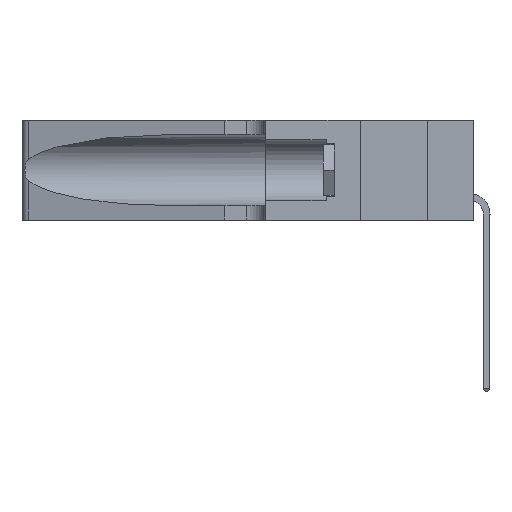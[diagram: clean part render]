
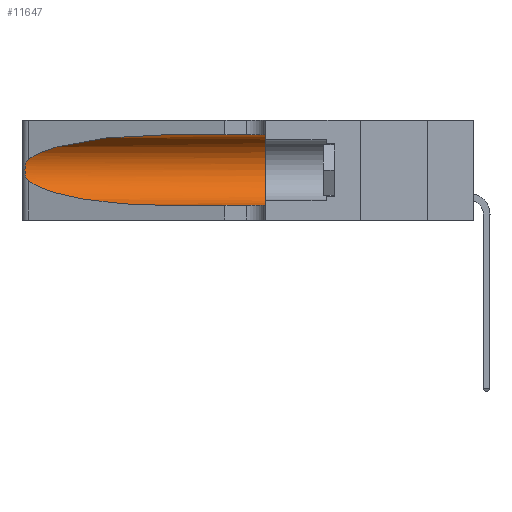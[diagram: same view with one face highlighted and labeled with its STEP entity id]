
A CAD part, left-side view. The second image highlights one B-rep face of the part: STEP entity #11647.
In plain terms, the highlighted cylindrical face has radius 3.308 mm (diameter 6.617 mm), a partial arc.
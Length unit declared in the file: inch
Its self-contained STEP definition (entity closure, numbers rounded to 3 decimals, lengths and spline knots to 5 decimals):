
#360 = EDGE_CURVE ( 'NONE', #12610, #28026, #2224, .T. ) ;
#1036 = CARTESIAN_POINT ( 'NONE',  ( 0.25639, 1.23184, 0.21858 ) ) ;
#2037 = AXIS2_PLACEMENT_3D ( 'NONE', #21559, #14705, #48827 ) ;
#2224 = CIRCLE ( 'NONE', #18384, 0.13025 ) ;
#2693 = CARTESIAN_POINT ( 'NONE',  ( 0.2373, 1.15595, 0.28018 ) ) ;
#3756 = VERTEX_POINT ( 'NONE', #14707 ) ;
#6056 = FACE_OUTER_BOUND ( 'NONE', #37666, .T. ) ;
#6677 = CARTESIAN_POINT ( 'NONE',  ( 0.18966, 0.96281, 0.31525 ) ) ;
#8108 = EDGE_CURVE ( 'NONE', #3756, #28026, #24553, .T. ) ;
#8240 = CARTESIAN_POINT ( 'NONE',  ( 0.25639, 1.23186, 0.15144 ) ) ;
#8394 = CARTESIAN_POINT ( 'NONE',  ( 0.1305, 0.35, 0.31525 ) ) ;
#8759 = CARTESIAN_POINT ( 'NONE',  ( 0.2373, 1.15595, 0.08982 ) ) ;
#11647 = ADVANCED_FACE ( 'NONE', ( #6056 ), #13809, .F. ) ;
#11880 = VERTEX_POINT ( 'NONE', #24815 ) ;
#11924 = CARTESIAN_POINT ( 'NONE',  ( 0.25854, 1.2359, 0.20912 ) ) ;
#12003 = DIRECTION ( 'NONE',  ( 0., -1., 0. ) ) ;
#12610 = VERTEX_POINT ( 'NONE', #8394 ) ;
#13329 = ORIENTED_EDGE ( 'NONE', *, *, #45015, .F. ) ;
#13809 = CYLINDRICAL_SURFACE ( 'NONE', #2037, 0.13025 ) ;
#14033 = B_SPLINE_CURVE_WITH_KNOTS ( 'NONE', 3,
 ( #19439, #45797, #1036, #16199, #11924, #20214, #23894, #38654, #46514, #27074, #42968, #8240, #31607, #34956 ),
 .UNSPECIFIED., .F., .F.,
 ( 4, 2, 2, 2, 2, 2, 4 ),
 ( 0., 0.00027, 0.00053, 0.00107, 0.0016, 0.00187, 0.00214 ),
 .UNSPECIFIED. ) ;
#14705 = DIRECTION ( 'NONE',  ( 0., -1., 0. ) ) ;
#14707 = CARTESIAN_POINT ( 'NONE',  ( 0.1305, 0.72297, 0.05475 ) ) ;
#16199 = CARTESIAN_POINT ( 'NONE',  ( 0.25787, 1.23484, 0.2124 ) ) ;
#16673 = CARTESIAN_POINT ( 'NONE',  ( 0.1305, 1.61858, 0.31525 ) ) ;
#18384 = AXIS2_PLACEMENT_3D ( 'NONE', #45486, #45820, #48797 ) ;
#19439 = CARTESIAN_POINT ( 'NONE',  ( 0.25487, 1.22718, 0.22369 ) ) ;
#20214 = CARTESIAN_POINT ( 'NONE',  ( 0.26018, 1.23835, 0.19895 ) ) ;
#21304 = EDGE_CURVE ( 'NONE', #37774, #3756, #41562, .T. ) ;
#21526 = CARTESIAN_POINT ( 'NONE',  ( 0.1305, 0.72297, 0.31525 ) ) ;
#21559 = CARTESIAN_POINT ( 'NONE',  ( 0.1305, 1.61858, 0.185 ) ) ;
#23354 = VECTOR ( 'NONE', #12003, 39.37008 ) ;
#23894 = CARTESIAN_POINT ( 'NONE',  ( 0.26075, 1.23896, 0.19203 ) ) ;
#24553 = LINE ( 'NONE', #35525, #23354 ) ;
#24815 = CARTESIAN_POINT ( 'NONE',  ( 0.1305, 0.72297, 0.31525 ) ) ;
#26564 = EDGE_CURVE ( 'NONE', #44749, #37774, #14033, .T. ) ;
#27074 = CARTESIAN_POINT ( 'NONE',  ( 0.25856, 1.23593, 0.16098 ) ) ;
#28026 = VERTEX_POINT ( 'NONE', #30961 ) ;
#28462 = VECTOR ( 'NONE', #35425, 39.37008 ) ;
#29386 = CARTESIAN_POINT ( 'NONE',  ( 0.25487, 1.22718, 0.14631 ) ) ;
#29561 = CARTESIAN_POINT ( 'NONE',  ( 0.25487, 1.22718, 0.22369 ) ) ;
#30186 = ORIENTED_EDGE ( 'NONE', *, *, #26564, .T. ) ;
#30636 = CARTESIAN_POINT ( 'NONE',  ( 0.25487, 1.22718, 0.22369 ) ) ;
#30961 = CARTESIAN_POINT ( 'NONE',  ( 0.1305, 0.35, 0.05475 ) ) ;
#31607 = CARTESIAN_POINT ( 'NONE',  ( 0.25555, 1.22993, 0.14849 ) ) ;
#34956 = CARTESIAN_POINT ( 'NONE',  ( 0.25487, 1.22718, 0.14631 ) ) ;
#35425 = DIRECTION ( 'NONE',  ( 0., -1., 0. ) ) ;
#35525 = CARTESIAN_POINT ( 'NONE',  ( 0.1305, 1.61858, 0.05475 ) ) ;
#37666 = EDGE_LOOP ( 'NONE', ( #45530, #30186, #45856, #41888, #42505, #13329 ) ) ;
#37774 = VERTEX_POINT ( 'NONE', #29386 ) ;
#38654 = CARTESIAN_POINT ( 'NONE',  ( 0.26075, 1.23896, 0.178 ) ) ;
#41562 =( BOUNDED_CURVE ( )  B_SPLINE_CURVE ( 3, ( #49454, #8759, #47016, #42528 ),
 .UNSPECIFIED., .F., .F. ) 
 B_SPLINE_CURVE_WITH_KNOTS ( ( 4, 4 ),
 ( 3.44316, 4.71239 ),
 .UNSPECIFIED. ) 
 CURVE ( )  GEOMETRIC_REPRESENTATION_ITEM ( )  RATIONAL_B_SPLINE_CURVE ( ( 1., 0.87, 0.87, 1. ) ) 
 REPRESENTATION_ITEM ( '' )  );
#41888 = ORIENTED_EDGE ( 'NONE', *, *, #8108, .T. ) ;
#42505 = ORIENTED_EDGE ( 'NONE', *, *, #360, .F. ) ;
#42528 = CARTESIAN_POINT ( 'NONE',  ( 0.1305, 0.72297, 0.05475 ) ) ;
#42778 =( BOUNDED_CURVE ( )  B_SPLINE_CURVE ( 3, ( #21526, #6677, #2693, #29561 ),
 .UNSPECIFIED., .F., .F. ) 
 B_SPLINE_CURVE_WITH_KNOTS ( ( 4, 4 ),
 ( 1.5708, 2.84003 ),
 .UNSPECIFIED. ) 
 CURVE ( )  GEOMETRIC_REPRESENTATION_ITEM ( )  RATIONAL_B_SPLINE_CURVE ( ( 1., 0.87, 0.87, 1. ) ) 
 REPRESENTATION_ITEM ( '' )  );
#42968 = CARTESIAN_POINT ( 'NONE',  ( 0.25789, 1.23486, 0.15765 ) ) ;
#43408 = LINE ( 'NONE', #16673, #28462 ) ;
#44749 = VERTEX_POINT ( 'NONE', #30636 ) ;
#45015 = EDGE_CURVE ( 'NONE', #11880, #12610, #43408, .T. ) ;
#45486 = CARTESIAN_POINT ( 'NONE',  ( 0.1305, 0.35, 0.185 ) ) ;
#45530 = ORIENTED_EDGE ( 'NONE', *, *, #45861, .T. ) ;
#45797 = CARTESIAN_POINT ( 'NONE',  ( 0.25555, 1.22994, 0.2215 ) ) ;
#45820 = DIRECTION ( 'NONE',  ( 0., 1., 0. ) ) ;
#45856 = ORIENTED_EDGE ( 'NONE', *, *, #21304, .T. ) ;
#45861 = EDGE_CURVE ( 'NONE', #11880, #44749, #42778, .T. ) ;
#46514 = CARTESIAN_POINT ( 'NONE',  ( 0.26017, 1.23833, 0.17102 ) ) ;
#47016 = CARTESIAN_POINT ( 'NONE',  ( 0.18966, 0.96281, 0.05475 ) ) ;
#48797 = DIRECTION ( 'NONE',  ( 0., 0., 1. ) ) ;
#48827 = DIRECTION ( 'NONE',  ( 0., 0., -1. ) ) ;
#49454 = CARTESIAN_POINT ( 'NONE',  ( 0.25487, 1.22718, 0.14631 ) ) ;
